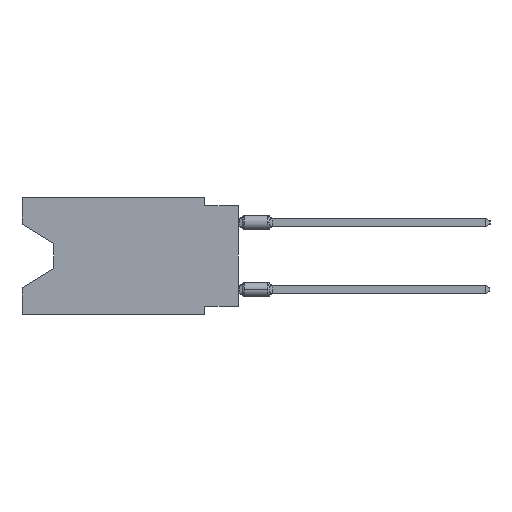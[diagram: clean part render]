
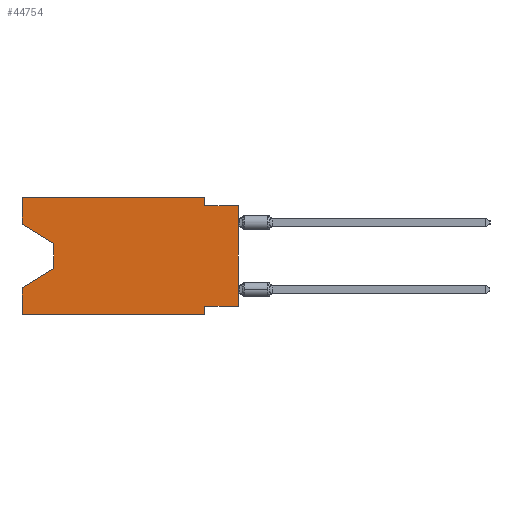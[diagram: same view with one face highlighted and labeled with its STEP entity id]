
A CAD part, left-side view. The second image highlights one B-rep face of the part: STEP entity #44754.
In plain terms, the highlighted planar face has unit normal (-1, 0, 0).
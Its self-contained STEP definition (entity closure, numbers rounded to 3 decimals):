
#1317 = CARTESIAN_POINT ( 'NONE',  ( 0., 16.383, -8.89 ) ) ;
#3553 = VERTEX_POINT ( 'NONE', #55060 ) ;
#3962 = FACE_OUTER_BOUND ( 'NONE', #24368, .T. ) ;
#4203 = CARTESIAN_POINT ( 'NONE',  ( 0., 13.97, -5.385 ) ) ;
#4306 = EDGE_CURVE ( 'NONE', #3553, #20122, #51059, .T. ) ;
#4457 = LINE ( 'NONE', #22051, #7388 ) ;
#5554 = EDGE_CURVE ( 'NONE', #56480, #36431, #19203, .T. ) ;
#6649 = DIRECTION ( 'NONE',  ( 0., 1., 0. ) ) ;
#7388 = VECTOR ( 'NONE', #39891, 1000. ) ;
#8642 = DIRECTION ( 'NONE',  ( 1., 0., 0. ) ) ;
#10284 = ORIENTED_EDGE ( 'NONE', *, *, #32187, .F. ) ;
#10420 = LINE ( 'NONE', #18910, #28525 ) ;
#10938 = CARTESIAN_POINT ( 'NONE',  ( 0., 13.97, -3.505 ) ) ;
#13659 = CARTESIAN_POINT ( 'NONE',  ( 0., 16.383, -2.038 ) ) ;
#14381 = VERTEX_POINT ( 'NONE', #55479 ) ;
#14463 = VECTOR ( 'NONE', #23689, 1000. ) ;
#16707 = CARTESIAN_POINT ( 'NONE',  ( 0., 16.383, 0. ) ) ;
#17048 = DIRECTION ( 'NONE',  ( 0., -0.855, -0.519 ) ) ;
#17330 = CARTESIAN_POINT ( 'NONE',  ( 0., 16.383, -2.038 ) ) ;
#17386 = CARTESIAN_POINT ( 'NONE',  ( 0., 16.383, 0. ) ) ;
#17441 = EDGE_CURVE ( 'NONE', #51374, #20122, #19834, .T. ) ;
#17581 = EDGE_CURVE ( 'NONE', #31539, #34904, #47357, .T. ) ;
#17633 = VECTOR ( 'NONE', #23357, 1000. ) ;
#18910 = CARTESIAN_POINT ( 'NONE',  ( 0., 2.54, 0. ) ) ;
#19203 = LINE ( 'NONE', #32647, #35516 ) ;
#19834 = LINE ( 'NONE', #37690, #17633 ) ;
#20055 = EDGE_CURVE ( 'NONE', #31539, #51374, #46754, .T. ) ;
#20116 = EDGE_CURVE ( 'NONE', #36431, #14381, #44590, .T. ) ;
#20122 = VERTEX_POINT ( 'NONE', #45451 ) ;
#20852 = ORIENTED_EDGE ( 'NONE', *, *, #5554, .T. ) ;
#22051 = CARTESIAN_POINT ( 'NONE',  ( 0., 16.383, 0. ) ) ;
#22337 = DIRECTION ( 'NONE',  ( 0., 0.855, -0.519 ) ) ;
#23112 = CARTESIAN_POINT ( 'NONE',  ( 0., 16.383, 0. ) ) ;
#23357 = DIRECTION ( 'NONE',  ( 0., 0., -1. ) ) ;
#23689 = DIRECTION ( 'NONE',  ( 0., 0., 1. ) ) ;
#23965 = LINE ( 'NONE', #32726, #47848 ) ;
#24368 = EDGE_LOOP ( 'NONE', ( #28770, #20852, #35179, #55522, #39794, #37826, #48423, #42954, #31818, #10284, #32830, #55185 ) ) ;
#25567 = EDGE_CURVE ( 'NONE', #52694, #52712, #4457, .T. ) ;
#25882 = LINE ( 'NONE', #17386, #29072 ) ;
#28525 = VECTOR ( 'NONE', #32944, 1000. ) ;
#28542 = DIRECTION ( 'NONE',  ( 0., -1., 0. ) ) ;
#28770 = ORIENTED_EDGE ( 'NONE', *, *, #28851, .T. ) ;
#28851 = EDGE_CURVE ( 'NONE', #34159, #56480, #41762, .T. ) ;
#29072 = VECTOR ( 'NONE', #48703, 1000. ) ;
#31539 = VERTEX_POINT ( 'NONE', #48881 ) ;
#31709 = EDGE_CURVE ( 'NONE', #34159, #52694, #46233, .T. ) ;
#31765 = CARTESIAN_POINT ( 'NONE',  ( 0., 2.54, -8.255 ) ) ;
#31818 = ORIENTED_EDGE ( 'NONE', *, *, #37816, .F. ) ;
#32187 = EDGE_CURVE ( 'NONE', #52712, #54779, #10420, .T. ) ;
#32647 = CARTESIAN_POINT ( 'NONE',  ( 0., 13.97, -3.505 ) ) ;
#32726 = CARTESIAN_POINT ( 'NONE',  ( 0., 0., -0.635 ) ) ;
#32830 = ORIENTED_EDGE ( 'NONE', *, *, #25567, .F. ) ;
#32944 = DIRECTION ( 'NONE',  ( 0., 0., -1. ) ) ;
#34159 = VERTEX_POINT ( 'NONE', #13659 ) ;
#34904 = VERTEX_POINT ( 'NONE', #36307 ) ;
#35179 = ORIENTED_EDGE ( 'NONE', *, *, #20116, .T. ) ;
#35391 = CARTESIAN_POINT ( 'NONE',  ( 0., 13.97, -5.385 ) ) ;
#35516 = VECTOR ( 'NONE', #49655, 1000. ) ;
#36307 = CARTESIAN_POINT ( 'NONE',  ( 0., 0., -0.635 ) ) ;
#36431 = VERTEX_POINT ( 'NONE', #35391 ) ;
#36535 = DIRECTION ( 'NONE',  ( 0., -1., 0. ) ) ;
#37420 = AXIS2_PLACEMENT_3D ( 'NONE', #39686, #8642, #53412 ) ;
#37619 = VECTOR ( 'NONE', #17048, 1000. ) ;
#37690 = CARTESIAN_POINT ( 'NONE',  ( 0., 2.54, -8.89 ) ) ;
#37816 = EDGE_CURVE ( 'NONE', #54779, #34904, #23965, .T. ) ;
#37826 = ORIENTED_EDGE ( 'NONE', *, *, #17441, .F. ) ;
#38341 = VECTOR ( 'NONE', #6649, 1000. ) ;
#39171 = EDGE_CURVE ( 'NONE', #3553, #14381, #25882, .T. ) ;
#39686 = CARTESIAN_POINT ( 'NONE',  ( 0., 16.383, 0. ) ) ;
#39794 = ORIENTED_EDGE ( 'NONE', *, *, #4306, .T. ) ;
#39891 = DIRECTION ( 'NONE',  ( 0., -1., 0. ) ) ;
#40085 = VECTOR ( 'NONE', #43230, 1000. ) ;
#41762 = LINE ( 'NONE', #17330, #37619 ) ;
#42954 = ORIENTED_EDGE ( 'NONE', *, *, #17581, .T. ) ;
#43230 = DIRECTION ( 'NONE',  ( 0., 0., 1. ) ) ;
#43353 = CARTESIAN_POINT ( 'NONE',  ( 0., 2.54, 0. ) ) ;
#44590 = LINE ( 'NONE', #4203, #57016 ) ;
#44754 = ADVANCED_FACE ( 'NONE', ( #3962 ), #48180, .F. ) ;
#45451 = CARTESIAN_POINT ( 'NONE',  ( 0., 2.54, -8.89 ) ) ;
#46233 = LINE ( 'NONE', #23112, #14463 ) ;
#46754 = LINE ( 'NONE', #56387, #38341 ) ;
#47357 = LINE ( 'NONE', #52010, #40085 ) ;
#47628 = CARTESIAN_POINT ( 'NONE',  ( 0., 2.54, -0.635 ) ) ;
#47848 = VECTOR ( 'NONE', #36535, 1000. ) ;
#48180 = PLANE ( 'NONE',  #37420 ) ;
#48423 = ORIENTED_EDGE ( 'NONE', *, *, #20055, .F. ) ;
#48489 = VECTOR ( 'NONE', #28542, 1000. ) ;
#48703 = DIRECTION ( 'NONE',  ( 0., 0., 1. ) ) ;
#48881 = CARTESIAN_POINT ( 'NONE',  ( 0., 0., -8.255 ) ) ;
#49655 = DIRECTION ( 'NONE',  ( 0., 0., -1. ) ) ;
#51059 = LINE ( 'NONE', #1317, #48489 ) ;
#51374 = VERTEX_POINT ( 'NONE', #31765 ) ;
#52010 = CARTESIAN_POINT ( 'NONE',  ( 0., 0., 0. ) ) ;
#52694 = VERTEX_POINT ( 'NONE', #16707 ) ;
#52712 = VERTEX_POINT ( 'NONE', #43353 ) ;
#53412 = DIRECTION ( 'NONE',  ( 0., 0., -1. ) ) ;
#54779 = VERTEX_POINT ( 'NONE', #47628 ) ;
#55060 = CARTESIAN_POINT ( 'NONE',  ( 0., 16.383, -8.89 ) ) ;
#55185 = ORIENTED_EDGE ( 'NONE', *, *, #31709, .F. ) ;
#55479 = CARTESIAN_POINT ( 'NONE',  ( 0., 16.383, -6.852 ) ) ;
#55522 = ORIENTED_EDGE ( 'NONE', *, *, #39171, .F. ) ;
#56387 = CARTESIAN_POINT ( 'NONE',  ( 0., 0., -8.255 ) ) ;
#56480 = VERTEX_POINT ( 'NONE', #10938 ) ;
#57016 = VECTOR ( 'NONE', #22337, 1000. ) ;
